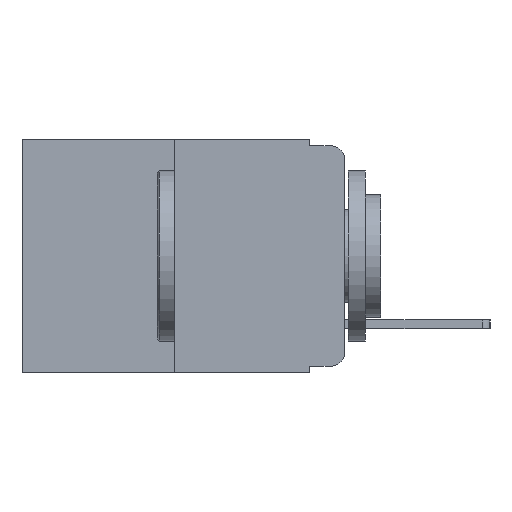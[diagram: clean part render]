
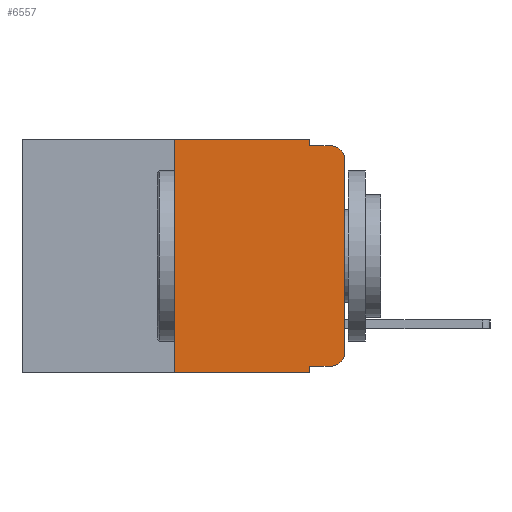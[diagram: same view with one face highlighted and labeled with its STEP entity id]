
A CAD part, left-side view. The second image highlights one B-rep face of the part: STEP entity #6557.
In plain terms, the highlighted planar face has unit normal (-1, 0, 0).
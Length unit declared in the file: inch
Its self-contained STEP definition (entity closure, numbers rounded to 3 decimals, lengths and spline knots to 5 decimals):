
#161 = PLANE ( 'NONE',  #3027 ) ;
#599 = DIRECTION ( 'NONE',  ( 0., -1., 0. ) ) ;
#621 = ORIENTED_EDGE ( 'NONE', *, *, #7637, .T. ) ;
#743 = VERTEX_POINT ( 'NONE', #6434 ) ;
#824 = LINE ( 'NONE', #8711, #5819 ) ;
#847 = CARTESIAN_POINT ( 'NONE',  ( 0., 0.051, 0. ) ) ;
#904 = CARTESIAN_POINT ( 'NONE',  ( 0., 0.25, 0. ) ) ;
#1052 = CARTESIAN_POINT ( 'NONE',  ( 0., 0.25, -0.343 ) ) ;
#1189 = DIRECTION ( 'NONE',  ( 1., 0., 0. ) ) ;
#1246 = ORIENTED_EDGE ( 'NONE', *, *, #3777, .F. ) ;
#1474 = CIRCLE ( 'NONE', #2794, 0.02 ) ;
#1588 = CARTESIAN_POINT ( 'NONE',  ( 0., 0.473, 0. ) ) ;
#1704 = LINE ( 'NONE', #1588, #4365 ) ;
#1706 = CARTESIAN_POINT ( 'NONE',  ( 0., 0.051, -0.343 ) ) ;
#1744 = CARTESIAN_POINT ( 'NONE',  ( 0., 0.051, 0. ) ) ;
#1856 = LINE ( 'NONE', #904, #6760 ) ;
#1903 = VECTOR ( 'NONE', #5066, 39.37008 ) ;
#1982 = VERTEX_POINT ( 'NONE', #3845 ) ;
#2009 = DIRECTION ( 'NONE',  ( -1., 0., 0. ) ) ;
#2234 = LINE ( 'NONE', #2759, #4553 ) ;
#2418 = LINE ( 'NONE', #1744, #3051 ) ;
#2705 = AXIS2_PLACEMENT_3D ( 'NONE', #7795, #2009, #8768 ) ;
#2759 = CARTESIAN_POINT ( 'NONE',  ( 0., 0., 0. ) ) ;
#2794 = AXIS2_PLACEMENT_3D ( 'NONE', #3303, #9927, #4288 ) ;
#3027 = AXIS2_PLACEMENT_3D ( 'NONE', #4165, #1189, #8003 ) ;
#3051 = VECTOR ( 'NONE', #8519, 39.37008 ) ;
#3303 = CARTESIAN_POINT ( 'NONE',  ( 0., 0.02, -0.313 ) ) ;
#3432 = CARTESIAN_POINT ( 'NONE',  ( 0., 0., -0.313 ) ) ;
#3565 = VERTEX_POINT ( 'NONE', #3432 ) ;
#3613 = ORIENTED_EDGE ( 'NONE', *, *, #6788, .F. ) ;
#3777 = EDGE_CURVE ( 'NONE', #5598, #6899, #2418, .T. ) ;
#3845 = CARTESIAN_POINT ( 'NONE',  ( 0., 0.02, -0.01 ) ) ;
#3954 = EDGE_LOOP ( 'NONE', ( #5614, #621, #5917, #10845, #3613, #6216, #11134, #1246, #6780, #9535 ) ) ;
#4165 = CARTESIAN_POINT ( 'NONE',  ( 0., 0.473, 0. ) ) ;
#4220 = VERTEX_POINT ( 'NONE', #5358 ) ;
#4288 = DIRECTION ( 'NONE',  ( 0., 0., -1. ) ) ;
#4365 = VECTOR ( 'NONE', #8374, 39.37008 ) ;
#4460 = EDGE_CURVE ( 'NONE', #3565, #11026, #2234, .T. ) ;
#4519 = FACE_OUTER_BOUND ( 'NONE', #3954, .T. ) ;
#4553 = VECTOR ( 'NONE', #4725, 39.37008 ) ;
#4725 = DIRECTION ( 'NONE',  ( 0., 0., 1. ) ) ;
#4958 = CIRCLE ( 'NONE', #2705, 0.02 ) ;
#5066 = DIRECTION ( 'NONE',  ( 0., -1., 0. ) ) ;
#5358 = CARTESIAN_POINT ( 'NONE',  ( 0., 0.051, 0. ) ) ;
#5575 = CARTESIAN_POINT ( 'NONE',  ( 0., 0.051, -0.333 ) ) ;
#5583 = EDGE_CURVE ( 'NONE', #5598, #743, #10255, .T. ) ;
#5598 = VERTEX_POINT ( 'NONE', #12090 ) ;
#5614 = ORIENTED_EDGE ( 'NONE', *, *, #4460, .T. ) ;
#5819 = VECTOR ( 'NONE', #12358, 39.37008 ) ;
#5917 = ORIENTED_EDGE ( 'NONE', *, *, #11357, .F. ) ;
#6051 = CARTESIAN_POINT ( 'NONE',  ( 0., 0.051, -0.01 ) ) ;
#6216 = ORIENTED_EDGE ( 'NONE', *, *, #6994, .F. ) ;
#6246 = VERTEX_POINT ( 'NONE', #8469 ) ;
#6434 = CARTESIAN_POINT ( 'NONE',  ( 0., 0.02, -0.333 ) ) ;
#6557 = ADVANCED_FACE ( 'NONE', ( #4519 ), #161, .F. ) ;
#6760 = VECTOR ( 'NONE', #8689, 39.37008 ) ;
#6780 = ORIENTED_EDGE ( 'NONE', *, *, #5583, .T. ) ;
#6788 = EDGE_CURVE ( 'NONE', #9880, #4220, #1704, .T. ) ;
#6899 = VERTEX_POINT ( 'NONE', #1706 ) ;
#6964 = LINE ( 'NONE', #847, #9162 ) ;
#6994 = EDGE_CURVE ( 'NONE', #10806, #9880, #1856, .T. ) ;
#7085 = LINE ( 'NONE', #6051, #1903 ) ;
#7262 = CARTESIAN_POINT ( 'NONE',  ( 0., 0., -0.03 ) ) ;
#7637 = EDGE_CURVE ( 'NONE', #11026, #1982, #4958, .T. ) ;
#7795 = CARTESIAN_POINT ( 'NONE',  ( 0., 0.02, -0.03 ) ) ;
#8003 = DIRECTION ( 'NONE',  ( 0., 0., -1. ) ) ;
#8374 = DIRECTION ( 'NONE',  ( 0., -1., 0. ) ) ;
#8469 = CARTESIAN_POINT ( 'NONE',  ( 0., 0.051, -0.01 ) ) ;
#8519 = DIRECTION ( 'NONE',  ( 0., 0., -1. ) ) ;
#8689 = DIRECTION ( 'NONE',  ( 0., 0., 1. ) ) ;
#8711 = CARTESIAN_POINT ( 'NONE',  ( 0., 0.473, -0.343 ) ) ;
#8768 = DIRECTION ( 'NONE',  ( 0., 0., -1. ) ) ;
#9162 = VECTOR ( 'NONE', #9499, 39.37008 ) ;
#9164 = EDGE_CURVE ( 'NONE', #743, #3565, #1474, .T. ) ;
#9499 = DIRECTION ( 'NONE',  ( 0., 0., -1. ) ) ;
#9535 = ORIENTED_EDGE ( 'NONE', *, *, #9164, .T. ) ;
#9880 = VERTEX_POINT ( 'NONE', #12044 ) ;
#9927 = DIRECTION ( 'NONE',  ( -1., 0., 0. ) ) ;
#10255 = LINE ( 'NONE', #5575, #12411 ) ;
#10806 = VERTEX_POINT ( 'NONE', #1052 ) ;
#10845 = ORIENTED_EDGE ( 'NONE', *, *, #11968, .F. ) ;
#11026 = VERTEX_POINT ( 'NONE', #7262 ) ;
#11134 = ORIENTED_EDGE ( 'NONE', *, *, #12047, .T. ) ;
#11357 = EDGE_CURVE ( 'NONE', #6246, #1982, #7085, .T. ) ;
#11968 = EDGE_CURVE ( 'NONE', #4220, #6246, #6964, .T. ) ;
#12044 = CARTESIAN_POINT ( 'NONE',  ( 0., 0.25, 0. ) ) ;
#12047 = EDGE_CURVE ( 'NONE', #10806, #6899, #824, .T. ) ;
#12090 = CARTESIAN_POINT ( 'NONE',  ( 0., 0.051, -0.333 ) ) ;
#12358 = DIRECTION ( 'NONE',  ( 0., -1., 0. ) ) ;
#12411 = VECTOR ( 'NONE', #599, 39.37008 ) ;
